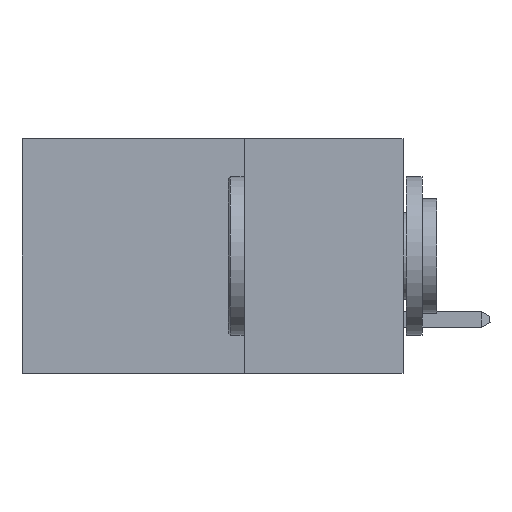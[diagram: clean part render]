
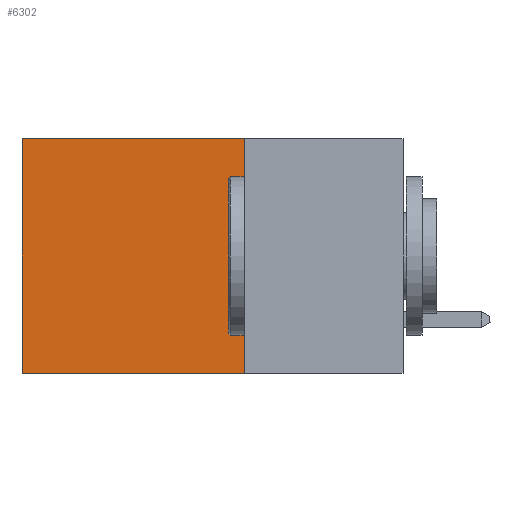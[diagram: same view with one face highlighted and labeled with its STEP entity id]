
A CAD part, left-side view. The second image highlights one B-rep face of the part: STEP entity #6302.
In plain terms, the highlighted planar face has unit normal (-1, 0, 0).
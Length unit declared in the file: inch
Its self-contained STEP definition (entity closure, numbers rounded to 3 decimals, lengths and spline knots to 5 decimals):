
#1487 = EDGE_CURVE ( 'NONE', #5695, #5405, #2704, .T. ) ;
#1498 = VECTOR ( 'NONE', #6025, 39.37008 ) ;
#1548 = LINE ( 'NONE', #7478, #8585 ) ;
#1963 = VECTOR ( 'NONE', #9428, 39.37008 ) ;
#1976 = EDGE_CURVE ( 'NONE', #10941, #11925, #10826, .T. ) ;
#2345 = CARTESIAN_POINT ( 'NONE',  ( 0.2875, 0.25, -0.37 ) ) ;
#2700 = EDGE_CURVE ( 'NONE', #5695, #10941, #1548, .T. ) ;
#2704 = LINE ( 'NONE', #2965, #8255 ) ;
#2965 = CARTESIAN_POINT ( 'NONE',  ( 0.2875, 0.25, 0. ) ) ;
#3618 = ORIENTED_EDGE ( 'NONE', *, *, #9429, .T. ) ;
#3631 = ORIENTED_EDGE ( 'NONE', *, *, #1976, .F. ) ;
#3668 = ORIENTED_EDGE ( 'NONE', *, *, #2700, .F. ) ;
#3672 = ORIENTED_EDGE ( 'NONE', *, *, #1487, .T. ) ;
#4227 = PLANE ( 'NONE',  #4448 ) ;
#4282 = EDGE_LOOP ( 'NONE', ( #3618, #3631, #3668, #3672 ) ) ;
#4448 = AXIS2_PLACEMENT_3D ( 'NONE', #10833, #13008, #6485 ) ;
#4558 = LINE ( 'NONE', #11471, #1498 ) ;
#5405 = VERTEX_POINT ( 'NONE', #13538 ) ;
#5695 = VERTEX_POINT ( 'NONE', #7475 ) ;
#6025 = DIRECTION ( 'NONE',  ( 0., 0., -1. ) ) ;
#6302 = ADVANCED_FACE ( 'NONE', ( #6568 ), #4227, .F. ) ;
#6485 = DIRECTION ( 'NONE',  ( 0., 0., -1. ) ) ;
#6497 = CARTESIAN_POINT ( 'NONE',  ( 0.2875, 0.25, -0.37 ) ) ;
#6568 = FACE_OUTER_BOUND ( 'NONE', #4282, .T. ) ;
#7475 = CARTESIAN_POINT ( 'NONE',  ( 0.2875, 0.25, 0. ) ) ;
#7478 = CARTESIAN_POINT ( 'NONE',  ( 0.2875, 0.25, 0. ) ) ;
#7689 = DIRECTION ( 'NONE',  ( 0., 0., -1. ) ) ;
#8255 = VECTOR ( 'NONE', #9118, 39.37008 ) ;
#8273 = CARTESIAN_POINT ( 'NONE',  ( 0.2875, 0.6, -0.37 ) ) ;
#8585 = VECTOR ( 'NONE', #7689, 39.37008 ) ;
#9118 = DIRECTION ( 'NONE',  ( 0., 1., 0. ) ) ;
#9428 = DIRECTION ( 'NONE',  ( 0., 1., 0. ) ) ;
#9429 = EDGE_CURVE ( 'NONE', #5405, #11925, #4558, .T. ) ;
#10826 = LINE ( 'NONE', #2345, #1963 ) ;
#10833 = CARTESIAN_POINT ( 'NONE',  ( 0.2875, 0.25, 0. ) ) ;
#10941 = VERTEX_POINT ( 'NONE', #6497 ) ;
#11471 = CARTESIAN_POINT ( 'NONE',  ( 0.2875, 0.6, 0. ) ) ;
#11925 = VERTEX_POINT ( 'NONE', #8273 ) ;
#13008 = DIRECTION ( 'NONE',  ( 1., 0., 0. ) ) ;
#13538 = CARTESIAN_POINT ( 'NONE',  ( 0.2875, 0.6, 0. ) ) ;
